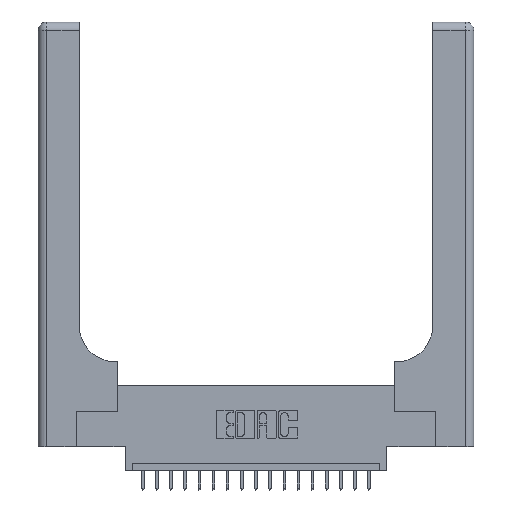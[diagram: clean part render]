
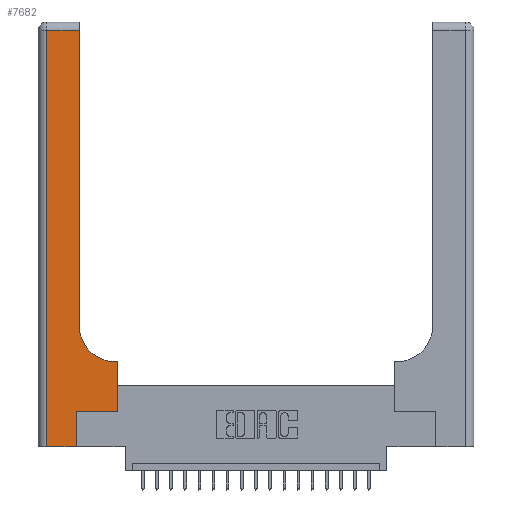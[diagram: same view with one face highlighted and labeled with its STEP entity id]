
A CAD part, top view. The second image highlights one B-rep face of the part: STEP entity #7682.
In plain terms, the highlighted planar face has unit normal (0, 0, 1).
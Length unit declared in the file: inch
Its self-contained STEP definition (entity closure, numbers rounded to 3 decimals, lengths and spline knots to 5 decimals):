
#236 = ORIENTED_EDGE ( 'NONE', *, *, #15971, .T. ) ;
#351 = DIRECTION ( 'NONE',  ( 0., 1., 0. ) ) ;
#651 = DIRECTION ( 'NONE',  ( 0., 0., -1. ) ) ;
#704 = CARTESIAN_POINT ( 'NONE',  ( 0.269, 0.25, 0.37 ) ) ;
#1610 = EDGE_CURVE ( 'NONE', #11629, #8320, #2340, .T. ) ;
#1801 = EDGE_CURVE ( 'NONE', #9004, #11629, #17144, .T. ) ;
#1899 = ORIENTED_EDGE ( 'NONE', *, *, #12202, .T. ) ;
#2210 = DIRECTION ( 'NONE',  ( 1., 0., 0. ) ) ;
#2304 = FACE_OUTER_BOUND ( 'NONE', #20631, .T. ) ;
#2340 = LINE ( 'NONE', #7337, #17965 ) ;
#2745 = ORIENTED_EDGE ( 'NONE', *, *, #6861, .T. ) ;
#2761 = VECTOR ( 'NONE', #5325, 39.37008 ) ;
#3366 = CARTESIAN_POINT ( 'NONE',  ( 0.5585, 0.25, 0.37 ) ) ;
#3461 = DIRECTION ( 'NONE',  ( 0., 1., 0. ) ) ;
#3510 = VECTOR ( 'NONE', #10971, 39.37008 ) ;
#3640 = EDGE_CURVE ( 'NONE', #8409, #9004, #15041, .T. ) ;
#3657 = EDGE_CURVE ( 'NONE', #15781, #19730, #13308, .T. ) ;
#4304 = LINE ( 'NONE', #704, #3510 ) ;
#4439 = DIRECTION ( 'NONE',  ( -1., 0., 0. ) ) ;
#5022 = VERTEX_POINT ( 'NONE', #13858 ) ;
#5112 = ORIENTED_EDGE ( 'NONE', *, *, #12734, .T. ) ;
#5325 = DIRECTION ( 'NONE',  ( -1., 0., 0. ) ) ;
#5566 = CARTESIAN_POINT ( 'NONE',  ( 0., 3., 0.37 ) ) ;
#6576 = CARTESIAN_POINT ( 'NONE',  ( 0.5585, 0.6, 0.37 ) ) ;
#6861 = EDGE_CURVE ( 'NONE', #21146, #8409, #10444, .T. ) ;
#7200 = CARTESIAN_POINT ( 'NONE',  ( 0., 0., 0.37 ) ) ;
#7337 = CARTESIAN_POINT ( 'NONE',  ( 0.269, 0., 0.37 ) ) ;
#7682 = ADVANCED_FACE ( 'NONE', ( #2304 ), #15611, .F. ) ;
#8135 = DIRECTION ( 'NONE',  ( 1., 0., 0. ) ) ;
#8320 = VERTEX_POINT ( 'NONE', #16662 ) ;
#8409 = VERTEX_POINT ( 'NONE', #18481 ) ;
#8503 = ORIENTED_EDGE ( 'NONE', *, *, #16780, .T. ) ;
#8679 = DIRECTION ( 'NONE',  ( 0., -1., 0. ) ) ;
#8687 = ORIENTED_EDGE ( 'NONE', *, *, #1801, .T. ) ;
#9004 = VERTEX_POINT ( 'NONE', #19312 ) ;
#10233 = CARTESIAN_POINT ( 'NONE',  ( 0., 2.94, 0.37 ) ) ;
#10386 = VECTOR ( 'NONE', #8679, 39.37008 ) ;
#10444 = LINE ( 'NONE', #10233, #2761 ) ;
#10835 = LINE ( 'NONE', #15319, #11618 ) ;
#10971 = DIRECTION ( 'NONE',  ( 1., 0., 0. ) ) ;
#11358 = CARTESIAN_POINT ( 'NONE',  ( 0.2915, 2.94, 0.37 ) ) ;
#11618 = VECTOR ( 'NONE', #351, 39.37008 ) ;
#11629 = VERTEX_POINT ( 'NONE', #16972 ) ;
#11856 = ORIENTED_EDGE ( 'NONE', *, *, #1610, .T. ) ;
#11994 = CARTESIAN_POINT ( 'NONE',  ( 0.5585, 0.25, 0.37 ) ) ;
#12202 = EDGE_CURVE ( 'NONE', #5022, #21146, #10835, .T. ) ;
#12228 = AXIS2_PLACEMENT_3D ( 'NONE', #5566, #651, #12459 ) ;
#12393 = DIRECTION ( 'NONE',  ( 0., 1., 0. ) ) ;
#12443 = VECTOR ( 'NONE', #2210, 39.37008 ) ;
#12459 = DIRECTION ( 'NONE',  ( -1., 0., 0. ) ) ;
#12734 = EDGE_CURVE ( 'NONE', #18283, #5022, #13373, .T. ) ;
#12849 = VECTOR ( 'NONE', #3461, 39.37008 ) ;
#13073 = DIRECTION ( 'NONE',  ( 0., 0., -1. ) ) ;
#13271 = VECTOR ( 'NONE', #4439, 39.37008 ) ;
#13308 = LINE ( 'NONE', #11994, #12849 ) ;
#13373 = CIRCLE ( 'NONE', #21003, 0.25 ) ;
#13858 = CARTESIAN_POINT ( 'NONE',  ( 0.2915, 0.85, 0.37 ) ) ;
#15041 = LINE ( 'NONE', #16985, #10386 ) ;
#15319 = CARTESIAN_POINT ( 'NONE',  ( 0.2915, 3., 0.37 ) ) ;
#15439 = CARTESIAN_POINT ( 'NONE',  ( 0.5415, 0.6, 0.37 ) ) ;
#15611 = PLANE ( 'NONE',  #12228 ) ;
#15781 = VERTEX_POINT ( 'NONE', #3366 ) ;
#15971 = EDGE_CURVE ( 'NONE', #19730, #18283, #16354, .T. ) ;
#16354 = LINE ( 'NONE', #21448, #13271 ) ;
#16450 = CARTESIAN_POINT ( 'NONE',  ( 0.5415, 0.85, 0.37 ) ) ;
#16662 = CARTESIAN_POINT ( 'NONE',  ( 0.269, 0.25, 0.37 ) ) ;
#16780 = EDGE_CURVE ( 'NONE', #8320, #15781, #4304, .T. ) ;
#16972 = CARTESIAN_POINT ( 'NONE',  ( 0.269, 0., 0.37 ) ) ;
#16985 = CARTESIAN_POINT ( 'NONE',  ( 0.06, 3., 0.37 ) ) ;
#17144 = LINE ( 'NONE', #7200, #12443 ) ;
#17931 = ORIENTED_EDGE ( 'NONE', *, *, #3657, .T. ) ;
#17965 = VECTOR ( 'NONE', #12393, 39.37008 ) ;
#18283 = VERTEX_POINT ( 'NONE', #15439 ) ;
#18481 = CARTESIAN_POINT ( 'NONE',  ( 0.06, 2.94, 0.37 ) ) ;
#19312 = CARTESIAN_POINT ( 'NONE',  ( 0.06, 0., 0.37 ) ) ;
#19730 = VERTEX_POINT ( 'NONE', #6576 ) ;
#20631 = EDGE_LOOP ( 'NONE', ( #1899, #2745, #20671, #8687, #11856, #8503, #17931, #236, #5112 ) ) ;
#20671 = ORIENTED_EDGE ( 'NONE', *, *, #3640, .T. ) ;
#21003 = AXIS2_PLACEMENT_3D ( 'NONE', #16450, #13073, #8135 ) ;
#21146 = VERTEX_POINT ( 'NONE', #11358 ) ;
#21448 = CARTESIAN_POINT ( 'NONE',  ( 0.2915, 0.6, 0.37 ) ) ;
